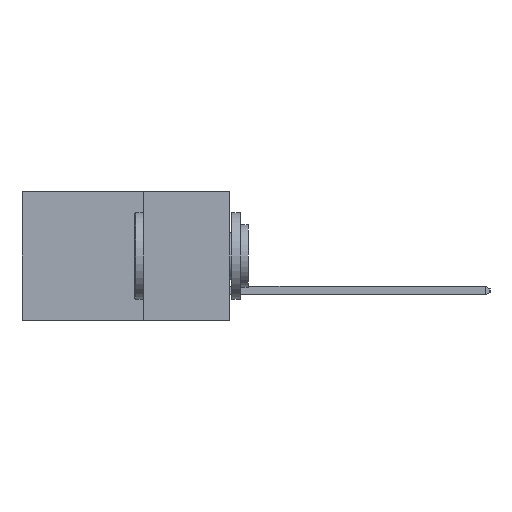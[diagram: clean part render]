
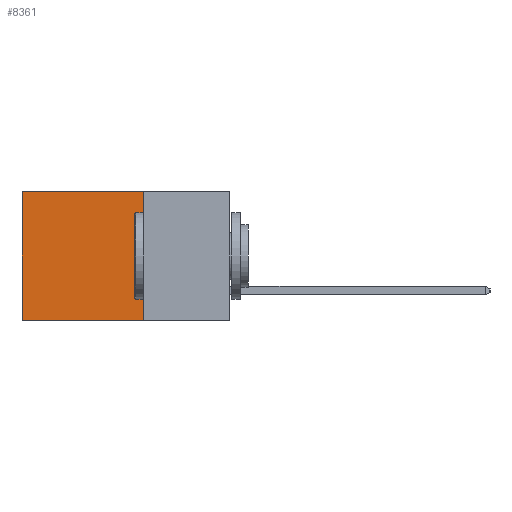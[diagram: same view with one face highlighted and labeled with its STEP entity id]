
A CAD part, left-side view. The second image highlights one B-rep face of the part: STEP entity #8361.
In plain terms, the highlighted planar face has unit normal (-1, 0, 0).
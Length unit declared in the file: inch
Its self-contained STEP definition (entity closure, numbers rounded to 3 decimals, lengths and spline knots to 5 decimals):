
#287 = CARTESIAN_POINT ( 'NONE',  ( 0.298, 0.6, -0.37 ) ) ;
#406 = ORIENTED_EDGE ( 'NONE', *, *, #5807, .F. ) ;
#408 = CARTESIAN_POINT ( 'NONE',  ( 0.298, 0.25, 0. ) ) ;
#1703 = LINE ( 'NONE', #10866, #5381 ) ;
#1817 = AXIS2_PLACEMENT_3D ( 'NONE', #408, #4331, #12150 ) ;
#1986 = DIRECTION ( 'NONE',  ( 0., 1., 0. ) ) ;
#2236 = CARTESIAN_POINT ( 'NONE',  ( 0.298, 0.25, -0.37 ) ) ;
#2386 = LINE ( 'NONE', #13477, #11142 ) ;
#2736 = EDGE_CURVE ( 'NONE', #11816, #8586, #2386, .T. ) ;
#3588 = DIRECTION ( 'NONE',  ( 0., 0., -1. ) ) ;
#4060 = VERTEX_POINT ( 'NONE', #10009 ) ;
#4331 = DIRECTION ( 'NONE',  ( 1., 0., 0. ) ) ;
#4373 = EDGE_CURVE ( 'NONE', #11816, #4060, #1703, .T. ) ;
#4430 = VECTOR ( 'NONE', #1986, 39.37008 ) ;
#4549 = LINE ( 'NONE', #8098, #10935 ) ;
#4983 = ORIENTED_EDGE ( 'NONE', *, *, #4373, .T. ) ;
#5196 = ORIENTED_EDGE ( 'NONE', *, *, #2736, .F. ) ;
#5381 = VECTOR ( 'NONE', #11040, 39.37008 ) ;
#5640 = VERTEX_POINT ( 'NONE', #287 ) ;
#5807 = EDGE_CURVE ( 'NONE', #8586, #5640, #7414, .T. ) ;
#5837 = EDGE_LOOP ( 'NONE', ( #9411, #406, #5196, #4983 ) ) ;
#6881 = CARTESIAN_POINT ( 'NONE',  ( 0.298, 0.25, -0.37 ) ) ;
#7414 = LINE ( 'NONE', #2236, #4430 ) ;
#7853 = FACE_OUTER_BOUND ( 'NONE', #5837, .T. ) ;
#8098 = CARTESIAN_POINT ( 'NONE',  ( 0.298, 0.6, 0. ) ) ;
#8361 = ADVANCED_FACE ( 'NONE', ( #7853 ), #10942, .F. ) ;
#8586 = VERTEX_POINT ( 'NONE', #6881 ) ;
#8653 = EDGE_CURVE ( 'NONE', #4060, #5640, #4549, .T. ) ;
#9411 = ORIENTED_EDGE ( 'NONE', *, *, #8653, .T. ) ;
#10009 = CARTESIAN_POINT ( 'NONE',  ( 0.298, 0.6, 0. ) ) ;
#10866 = CARTESIAN_POINT ( 'NONE',  ( 0.298, 0.25, 0. ) ) ;
#10935 = VECTOR ( 'NONE', #14794, 39.37008 ) ;
#10942 = PLANE ( 'NONE',  #1817 ) ;
#11040 = DIRECTION ( 'NONE',  ( 0., 1., 0. ) ) ;
#11142 = VECTOR ( 'NONE', #3588, 39.37008 ) ;
#11816 = VERTEX_POINT ( 'NONE', #14333 ) ;
#12150 = DIRECTION ( 'NONE',  ( 0., 0., -1. ) ) ;
#13477 = CARTESIAN_POINT ( 'NONE',  ( 0.298, 0.25, 0. ) ) ;
#14333 = CARTESIAN_POINT ( 'NONE',  ( 0.298, 0.25, 0. ) ) ;
#14794 = DIRECTION ( 'NONE',  ( 0., 0., -1. ) ) ;
